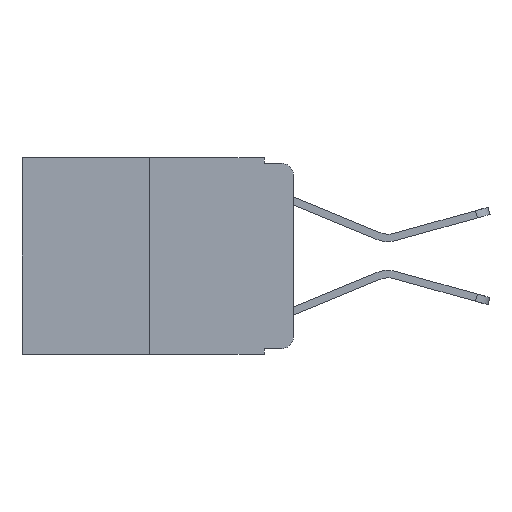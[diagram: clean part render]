
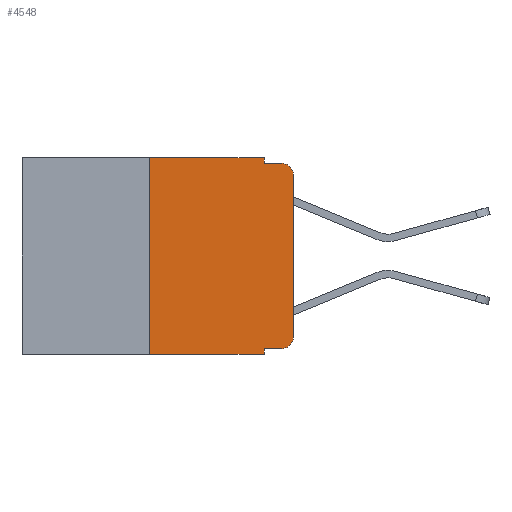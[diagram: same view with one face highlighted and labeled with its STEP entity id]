
A CAD part, left-side view. The second image highlights one B-rep face of the part: STEP entity #4548.
In plain terms, the highlighted planar face has unit normal (-1, 0, 0).
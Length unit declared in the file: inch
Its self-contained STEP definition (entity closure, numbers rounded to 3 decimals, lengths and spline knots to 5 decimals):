
#484 = VECTOR ( 'NONE', #13446, 39.37008 ) ;
#868 = EDGE_CURVE ( 'NONE', #18414, #10480, #14057, .T. ) ;
#1075 = CARTESIAN_POINT ( 'NONE',  ( 0., 0.25, 0. ) ) ;
#1277 = VECTOR ( 'NONE', #20678, 39.37008 ) ;
#1367 = DIRECTION ( 'NONE',  ( 0., 0., 1. ) ) ;
#3279 = EDGE_CURVE ( 'NONE', #16005, #19444, #13477, .T. ) ;
#3306 = CARTESIAN_POINT ( 'NONE',  ( 0., 0., 0. ) ) ;
#3646 = LINE ( 'NONE', #8907, #14047 ) ;
#3747 = EDGE_CURVE ( 'NONE', #6371, #13328, #23672, .T. ) ;
#3767 = ORIENTED_EDGE ( 'NONE', *, *, #22441, .T. ) ;
#4153 = CARTESIAN_POINT ( 'NONE',  ( 0., 0.051, -0.333 ) ) ;
#4188 = DIRECTION ( 'NONE',  ( 0., 0., -1. ) ) ;
#4418 = ORIENTED_EDGE ( 'NONE', *, *, #8996, .F. ) ;
#4548 = ADVANCED_FACE ( 'NONE', ( #20364 ), #10014, .F. ) ;
#4594 = CARTESIAN_POINT ( 'NONE',  ( 0., 0.051, -0.343 ) ) ;
#4881 = VERTEX_POINT ( 'NONE', #24516 ) ;
#5163 = CARTESIAN_POINT ( 'NONE',  ( 0., 0.02, -0.333 ) ) ;
#5718 = LINE ( 'NONE', #1075, #24496 ) ;
#6284 = AXIS2_PLACEMENT_3D ( 'NONE', #13944, #15901, #4188 ) ;
#6371 = VERTEX_POINT ( 'NONE', #15566 ) ;
#6934 = ORIENTED_EDGE ( 'NONE', *, *, #3279, .T. ) ;
#7070 = CARTESIAN_POINT ( 'NONE',  ( 0., 0.473, 0. ) ) ;
#7106 = EDGE_CURVE ( 'NONE', #9651, #10701, #16909, .T. ) ;
#7223 = DIRECTION ( 'NONE',  ( -1., 0., 0. ) ) ;
#8409 = VECTOR ( 'NONE', #19733, 39.37008 ) ;
#8845 = VECTOR ( 'NONE', #17170, 39.37008 ) ;
#8907 = CARTESIAN_POINT ( 'NONE',  ( 0., 0.051, 0. ) ) ;
#8957 = VECTOR ( 'NONE', #24589, 39.37008 ) ;
#8996 = EDGE_CURVE ( 'NONE', #18414, #9651, #5718, .T. ) ;
#9489 = CARTESIAN_POINT ( 'NONE',  ( 0., 0.051, 0. ) ) ;
#9651 = VERTEX_POINT ( 'NONE', #13802 ) ;
#10014 = PLANE ( 'NONE',  #6284 ) ;
#10046 = AXIS2_PLACEMENT_3D ( 'NONE', #18889, #7223, #20820 ) ;
#10480 = VERTEX_POINT ( 'NONE', #4594 ) ;
#10521 = ORIENTED_EDGE ( 'NONE', *, *, #23727, .F. ) ;
#10584 = DIRECTION ( 'NONE',  ( -1., 0., 0. ) ) ;
#10701 = VERTEX_POINT ( 'NONE', #9489 ) ;
#10899 = CARTESIAN_POINT ( 'NONE',  ( 0., 0.25, -0.343 ) ) ;
#11201 = CARTESIAN_POINT ( 'NONE',  ( 0., 0.473, -0.343 ) ) ;
#11479 = ORIENTED_EDGE ( 'NONE', *, *, #868, .T. ) ;
#11526 = ORIENTED_EDGE ( 'NONE', *, *, #18127, .T. ) ;
#13328 = VERTEX_POINT ( 'NONE', #21957 ) ;
#13446 = DIRECTION ( 'NONE',  ( 0., 0., -1. ) ) ;
#13477 = CIRCLE ( 'NONE', #16235, 0.02 ) ;
#13802 = CARTESIAN_POINT ( 'NONE',  ( 0., 0.25, 0. ) ) ;
#13944 = CARTESIAN_POINT ( 'NONE',  ( 0., 0.473, 0. ) ) ;
#14047 = VECTOR ( 'NONE', #22449, 39.37008 ) ;
#14057 = LINE ( 'NONE', #11201, #8845 ) ;
#14852 = VERTEX_POINT ( 'NONE', #20555 ) ;
#15566 = CARTESIAN_POINT ( 'NONE',  ( 0., 0., -0.03 ) ) ;
#15901 = DIRECTION ( 'NONE',  ( 1., 0., 0. ) ) ;
#16005 = VERTEX_POINT ( 'NONE', #5163 ) ;
#16235 = AXIS2_PLACEMENT_3D ( 'NONE', #22141, #10584, #24072 ) ;
#16844 = EDGE_CURVE ( 'NONE', #10701, #4881, #3646, .T. ) ;
#16909 = LINE ( 'NONE', #7070, #1277 ) ;
#17170 = DIRECTION ( 'NONE',  ( 0., -1., 0. ) ) ;
#17227 = ORIENTED_EDGE ( 'NONE', *, *, #3747, .T. ) ;
#18127 = EDGE_CURVE ( 'NONE', #14852, #16005, #23853, .T. ) ;
#18414 = VERTEX_POINT ( 'NONE', #10899 ) ;
#18597 = DIRECTION ( 'NONE',  ( 0., 0., 1. ) ) ;
#18754 = ORIENTED_EDGE ( 'NONE', *, *, #7106, .F. ) ;
#18853 = EDGE_LOOP ( 'NONE', ( #3767, #17227, #10521, #21443, #18754, #4418, #11479, #22973, #11526, #6934 ) ) ;
#18889 = CARTESIAN_POINT ( 'NONE',  ( 0., 0.02, -0.03 ) ) ;
#19206 = CARTESIAN_POINT ( 'NONE',  ( 0., 0.051, 0. ) ) ;
#19311 = LINE ( 'NONE', #22659, #8957 ) ;
#19444 = VERTEX_POINT ( 'NONE', #21835 ) ;
#19733 = DIRECTION ( 'NONE',  ( 0., -1., 0. ) ) ;
#20030 = VECTOR ( 'NONE', #1367, 39.37008 ) ;
#20364 = FACE_OUTER_BOUND ( 'NONE', #18853, .T. ) ;
#20555 = CARTESIAN_POINT ( 'NONE',  ( 0., 0.051, -0.333 ) ) ;
#20678 = DIRECTION ( 'NONE',  ( 0., -1., 0. ) ) ;
#20820 = DIRECTION ( 'NONE',  ( 0., 0., -1. ) ) ;
#21263 = LINE ( 'NONE', #19206, #484 ) ;
#21443 = ORIENTED_EDGE ( 'NONE', *, *, #16844, .F. ) ;
#21835 = CARTESIAN_POINT ( 'NONE',  ( 0., 0., -0.313 ) ) ;
#21957 = CARTESIAN_POINT ( 'NONE',  ( 0., 0.02, -0.01 ) ) ;
#21965 = EDGE_CURVE ( 'NONE', #14852, #10480, #21263, .T. ) ;
#22141 = CARTESIAN_POINT ( 'NONE',  ( 0., 0.02, -0.313 ) ) ;
#22441 = EDGE_CURVE ( 'NONE', #19444, #6371, #25105, .T. ) ;
#22449 = DIRECTION ( 'NONE',  ( 0., 0., -1. ) ) ;
#22659 = CARTESIAN_POINT ( 'NONE',  ( 0., 0.051, -0.01 ) ) ;
#22973 = ORIENTED_EDGE ( 'NONE', *, *, #21965, .F. ) ;
#23672 = CIRCLE ( 'NONE', #10046, 0.02 ) ;
#23727 = EDGE_CURVE ( 'NONE', #4881, #13328, #19311, .T. ) ;
#23853 = LINE ( 'NONE', #4153, #8409 ) ;
#24072 = DIRECTION ( 'NONE',  ( 0., 0., -1. ) ) ;
#24496 = VECTOR ( 'NONE', #18597, 39.37008 ) ;
#24516 = CARTESIAN_POINT ( 'NONE',  ( 0., 0.051, -0.01 ) ) ;
#24589 = DIRECTION ( 'NONE',  ( 0., -1., 0. ) ) ;
#25105 = LINE ( 'NONE', #3306, #20030 ) ;
